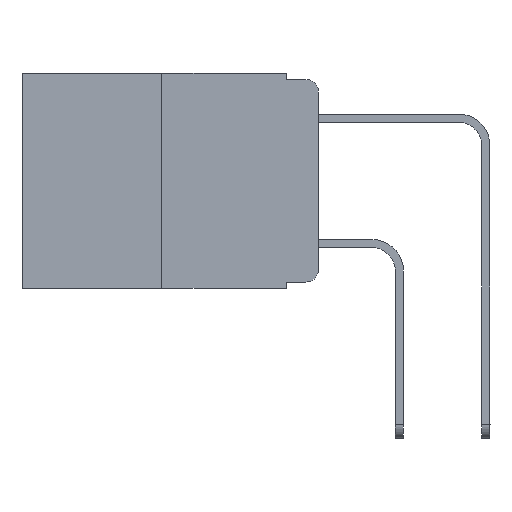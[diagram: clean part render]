
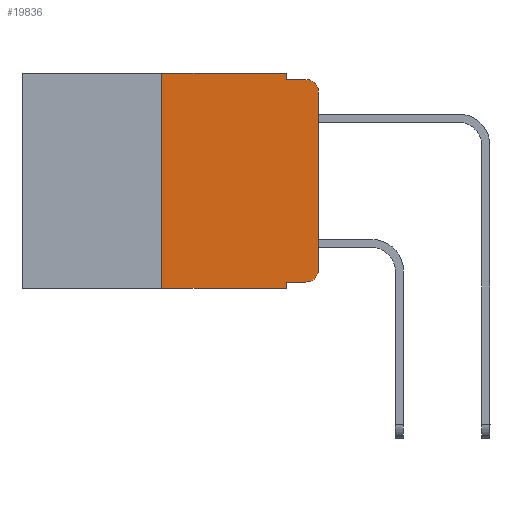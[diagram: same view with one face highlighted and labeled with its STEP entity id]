
A CAD part, left-side view. The second image highlights one B-rep face of the part: STEP entity #19836.
In plain terms, the highlighted planar face has unit normal (-1, 0, 0).
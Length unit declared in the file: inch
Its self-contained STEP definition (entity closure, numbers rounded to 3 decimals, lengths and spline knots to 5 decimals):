
#458 = CARTESIAN_POINT ( 'NONE',  ( 0., 0.051, -0.01 ) ) ;
#1212 = DIRECTION ( 'NONE',  ( -1., 0., 0. ) ) ;
#1352 = EDGE_CURVE ( 'NONE', #18932, #1549, #2967, .T. ) ;
#1549 = VERTEX_POINT ( 'NONE', #12559 ) ;
#1588 = EDGE_CURVE ( 'NONE', #21352, #8311, #14345, .T. ) ;
#2140 = ORIENTED_EDGE ( 'NONE', *, *, #4690, .T. ) ;
#2184 = LINE ( 'NONE', #9092, #8749 ) ;
#2868 = ORIENTED_EDGE ( 'NONE', *, *, #14863, .F. ) ;
#2967 = LINE ( 'NONE', #9871, #15573 ) ;
#3713 = DIRECTION ( 'NONE',  ( 0., 0., -1. ) ) ;
#3792 = EDGE_CURVE ( 'NONE', #16592, #9433, #11333, .T. ) ;
#3985 = CARTESIAN_POINT ( 'NONE',  ( 0., 0., 0. ) ) ;
#4185 = EDGE_CURVE ( 'NONE', #16592, #8965, #8162, .T. ) ;
#4298 = CARTESIAN_POINT ( 'NONE',  ( 0., 0.02, -0.03 ) ) ;
#4470 = CARTESIAN_POINT ( 'NONE',  ( 0., 0.25, 0. ) ) ;
#4690 = EDGE_CURVE ( 'NONE', #8311, #1549, #15369, .T. ) ;
#4959 = ORIENTED_EDGE ( 'NONE', *, *, #4185, .T. ) ;
#5412 = PLANE ( 'NONE',  #18073 ) ;
#5454 = ORIENTED_EDGE ( 'NONE', *, *, #9408, .T. ) ;
#5966 = VECTOR ( 'NONE', #14676, 39.37008 ) ;
#6138 = CARTESIAN_POINT ( 'NONE',  ( 0., 0., -0.313 ) ) ;
#6192 = AXIS2_PLACEMENT_3D ( 'NONE', #14769, #8015, #11401 ) ;
#6966 = DIRECTION ( 'NONE',  ( 0., -1., 0. ) ) ;
#7081 = DIRECTION ( 'NONE',  ( 0., 0., -1. ) ) ;
#8015 = DIRECTION ( 'NONE',  ( -1., 0., 0. ) ) ;
#8162 = LINE ( 'NONE', #14923, #21862 ) ;
#8311 = VERTEX_POINT ( 'NONE', #14868 ) ;
#8749 = VECTOR ( 'NONE', #7081, 39.37008 ) ;
#8965 = VERTEX_POINT ( 'NONE', #19348 ) ;
#9092 = CARTESIAN_POINT ( 'NONE',  ( 0., 0.051, 0. ) ) ;
#9342 = CARTESIAN_POINT ( 'NONE',  ( 0., 0.051, -0.333 ) ) ;
#9365 = ORIENTED_EDGE ( 'NONE', *, *, #20326, .T. ) ;
#9408 = EDGE_CURVE ( 'NONE', #22196, #19266, #14523, .T. ) ;
#9433 = VERTEX_POINT ( 'NONE', #10928 ) ;
#9871 = CARTESIAN_POINT ( 'NONE',  ( 0., 0.051, -0.01 ) ) ;
#9904 = LINE ( 'NONE', #15082, #19686 ) ;
#9928 = EDGE_CURVE ( 'NONE', #22110, #18932, #19181, .T. ) ;
#10116 = ORIENTED_EDGE ( 'NONE', *, *, #1588, .T. ) ;
#10119 = CARTESIAN_POINT ( 'NONE',  ( 0., 0.051, -0.333 ) ) ;
#10928 = CARTESIAN_POINT ( 'NONE',  ( 0., 0.25, 0. ) ) ;
#11333 = LINE ( 'NONE', #4470, #22346 ) ;
#11401 = DIRECTION ( 'NONE',  ( 0., 0., -1. ) ) ;
#11677 = DIRECTION ( 'NONE',  ( 0., -1., 0. ) ) ;
#12071 = ORIENTED_EDGE ( 'NONE', *, *, #16086, .F. ) ;
#12279 = DIRECTION ( 'NONE',  ( 1., 0., 0. ) ) ;
#12281 = EDGE_LOOP ( 'NONE', ( #10116, #2140, #20308, #16639, #12071, #17115, #4959, #2868, #5454, #9365 ) ) ;
#12559 = CARTESIAN_POINT ( 'NONE',  ( 0., 0.02, -0.01 ) ) ;
#12975 = DIRECTION ( 'NONE',  ( 0., 0., -1. ) ) ;
#14345 = LINE ( 'NONE', #3985, #5966 ) ;
#14523 = LINE ( 'NONE', #9342, #22372 ) ;
#14676 = DIRECTION ( 'NONE',  ( 0., 0., 1. ) ) ;
#14769 = CARTESIAN_POINT ( 'NONE',  ( 0., 0.02, -0.313 ) ) ;
#14863 = EDGE_CURVE ( 'NONE', #22196, #8965, #2184, .T. ) ;
#14868 = CARTESIAN_POINT ( 'NONE',  ( 0., 0., -0.03 ) ) ;
#14923 = CARTESIAN_POINT ( 'NONE',  ( 0., 0.473, -0.343 ) ) ;
#15028 = CARTESIAN_POINT ( 'NONE',  ( 0., 0.02, -0.333 ) ) ;
#15060 = DIRECTION ( 'NONE',  ( 0., 0., 1. ) ) ;
#15082 = CARTESIAN_POINT ( 'NONE',  ( 0., 0.473, 0. ) ) ;
#15369 = CIRCLE ( 'NONE', #20444, 0.02 ) ;
#15573 = VECTOR ( 'NONE', #11677, 39.37008 ) ;
#16086 = EDGE_CURVE ( 'NONE', #9433, #22110, #9904, .T. ) ;
#16117 = DIRECTION ( 'NONE',  ( 0., -1., 0. ) ) ;
#16225 = CARTESIAN_POINT ( 'NONE',  ( 0., 0.051, 0. ) ) ;
#16592 = VERTEX_POINT ( 'NONE', #19886 ) ;
#16639 = ORIENTED_EDGE ( 'NONE', *, *, #9928, .F. ) ;
#16921 = VECTOR ( 'NONE', #19624, 39.37008 ) ;
#17115 = ORIENTED_EDGE ( 'NONE', *, *, #3792, .F. ) ;
#18073 = AXIS2_PLACEMENT_3D ( 'NONE', #20549, #12279, #3713 ) ;
#18932 = VERTEX_POINT ( 'NONE', #458 ) ;
#19181 = LINE ( 'NONE', #19402, #16921 ) ;
#19266 = VERTEX_POINT ( 'NONE', #15028 ) ;
#19348 = CARTESIAN_POINT ( 'NONE',  ( 0., 0.051, -0.343 ) ) ;
#19402 = CARTESIAN_POINT ( 'NONE',  ( 0., 0.051, 0. ) ) ;
#19624 = DIRECTION ( 'NONE',  ( 0., 0., -1. ) ) ;
#19686 = VECTOR ( 'NONE', #6966, 39.37008 ) ;
#19836 = ADVANCED_FACE ( 'NONE', ( #20882 ), #5412, .F. ) ;
#19886 = CARTESIAN_POINT ( 'NONE',  ( 0., 0.25, -0.343 ) ) ;
#20265 = DIRECTION ( 'NONE',  ( 0., -1., 0. ) ) ;
#20308 = ORIENTED_EDGE ( 'NONE', *, *, #1352, .F. ) ;
#20326 = EDGE_CURVE ( 'NONE', #19266, #21352, #21696, .T. ) ;
#20444 = AXIS2_PLACEMENT_3D ( 'NONE', #4298, #1212, #12975 ) ;
#20549 = CARTESIAN_POINT ( 'NONE',  ( 0., 0.473, 0. ) ) ;
#20882 = FACE_OUTER_BOUND ( 'NONE', #12281, .T. ) ;
#21352 = VERTEX_POINT ( 'NONE', #6138 ) ;
#21696 = CIRCLE ( 'NONE', #6192, 0.02 ) ;
#21862 = VECTOR ( 'NONE', #20265, 39.37008 ) ;
#22110 = VERTEX_POINT ( 'NONE', #16225 ) ;
#22196 = VERTEX_POINT ( 'NONE', #10119 ) ;
#22346 = VECTOR ( 'NONE', #15060, 39.37008 ) ;
#22372 = VECTOR ( 'NONE', #16117, 39.37008 ) ;
